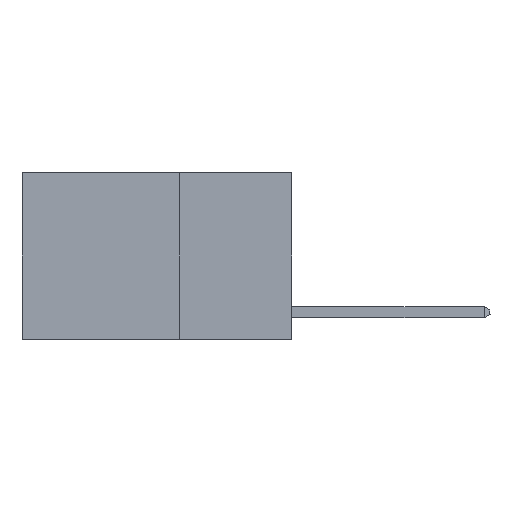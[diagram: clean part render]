
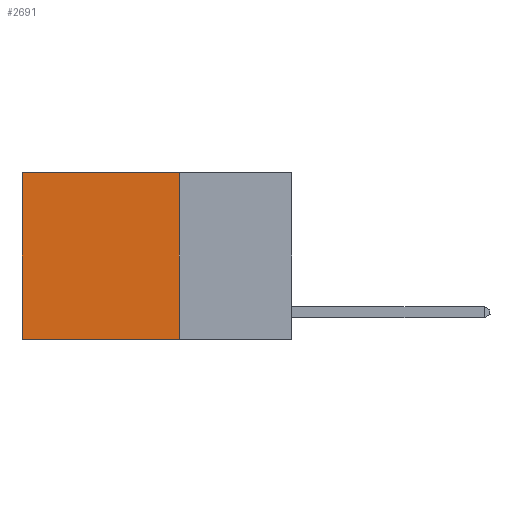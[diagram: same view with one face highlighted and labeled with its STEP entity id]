
A CAD part, left-side view. The second image highlights one B-rep face of the part: STEP entity #2691.
In plain terms, the highlighted planar face has unit normal (-1, 0, 0).
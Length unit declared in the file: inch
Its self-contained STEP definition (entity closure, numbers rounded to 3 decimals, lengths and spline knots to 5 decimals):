
#245 = CARTESIAN_POINT ( 'NONE',  ( 0.2625, 0.6, 0. ) ) ;
#282 = VERTEX_POINT ( 'NONE', #5509 ) ;
#639 = VERTEX_POINT ( 'NONE', #245 ) ;
#1210 = DIRECTION ( 'NONE',  ( 0., 0., -1. ) ) ;
#1351 = DIRECTION ( 'NONE',  ( 0., 1., 0. ) ) ;
#2691 = ADVANCED_FACE ( 'NONE', ( #21839 ), #12266, .F. ) ;
#2720 = ORIENTED_EDGE ( 'NONE', *, *, #20610, .F. ) ;
#4510 = ORIENTED_EDGE ( 'NONE', *, *, #5412, .T. ) ;
#4749 = CARTESIAN_POINT ( 'NONE',  ( 0.2625, 0.25, 0. ) ) ;
#5165 = CARTESIAN_POINT ( 'NONE',  ( 0.2625, 0.25, 0. ) ) ;
#5412 = EDGE_CURVE ( 'NONE', #639, #22841, #19883, .T. ) ;
#5509 = CARTESIAN_POINT ( 'NONE',  ( 0.2625, 0.25, 0. ) ) ;
#8479 = DIRECTION ( 'NONE',  ( 0., 0., -1. ) ) ;
#8674 = EDGE_CURVE ( 'NONE', #282, #639, #12423, .T. ) ;
#9433 = LINE ( 'NONE', #16923, #18360 ) ;
#10548 = LINE ( 'NONE', #18044, #23412 ) ;
#11054 = VECTOR ( 'NONE', #12552, 39.37008 ) ;
#11931 = VECTOR ( 'NONE', #1210, 39.37008 ) ;
#12157 = CARTESIAN_POINT ( 'NONE',  ( 0.2625, 0.6, 0. ) ) ;
#12266 = PLANE ( 'NONE',  #14814 ) ;
#12423 = LINE ( 'NONE', #5165, #11054 ) ;
#12552 = DIRECTION ( 'NONE',  ( 0., 1., 0. ) ) ;
#14174 = CARTESIAN_POINT ( 'NONE',  ( 0.2625, 0.6, -0.37 ) ) ;
#14814 = AXIS2_PLACEMENT_3D ( 'NONE', #4749, #15838, #8479 ) ;
#15425 = EDGE_LOOP ( 'NONE', ( #4510, #2720, #17690, #18115 ) ) ;
#15838 = DIRECTION ( 'NONE',  ( 1., 0., 0. ) ) ;
#16631 = VERTEX_POINT ( 'NONE', #23216 ) ;
#16923 = CARTESIAN_POINT ( 'NONE',  ( 0.2625, 0.25, 0. ) ) ;
#17045 = DIRECTION ( 'NONE',  ( 0., 0., -1. ) ) ;
#17690 = ORIENTED_EDGE ( 'NONE', *, *, #21921, .F. ) ;
#18044 = CARTESIAN_POINT ( 'NONE',  ( 0.2625, 0.25, -0.37 ) ) ;
#18115 = ORIENTED_EDGE ( 'NONE', *, *, #8674, .T. ) ;
#18360 = VECTOR ( 'NONE', #17045, 39.37008 ) ;
#19883 = LINE ( 'NONE', #12157, #11931 ) ;
#20610 = EDGE_CURVE ( 'NONE', #16631, #22841, #10548, .T. ) ;
#21839 = FACE_OUTER_BOUND ( 'NONE', #15425, .T. ) ;
#21921 = EDGE_CURVE ( 'NONE', #282, #16631, #9433, .T. ) ;
#22841 = VERTEX_POINT ( 'NONE', #14174 ) ;
#23216 = CARTESIAN_POINT ( 'NONE',  ( 0.2625, 0.25, -0.37 ) ) ;
#23412 = VECTOR ( 'NONE', #1351, 39.37008 ) ;
